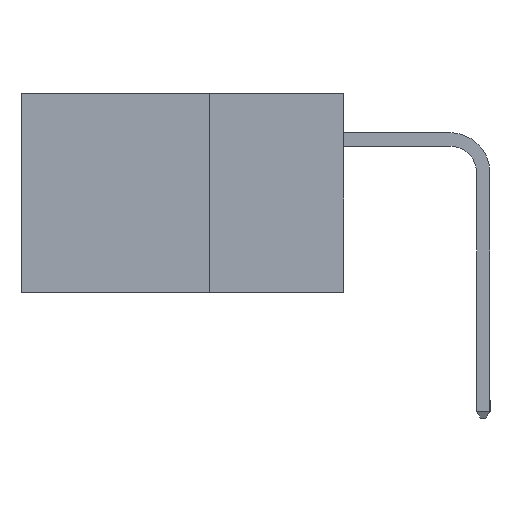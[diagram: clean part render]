
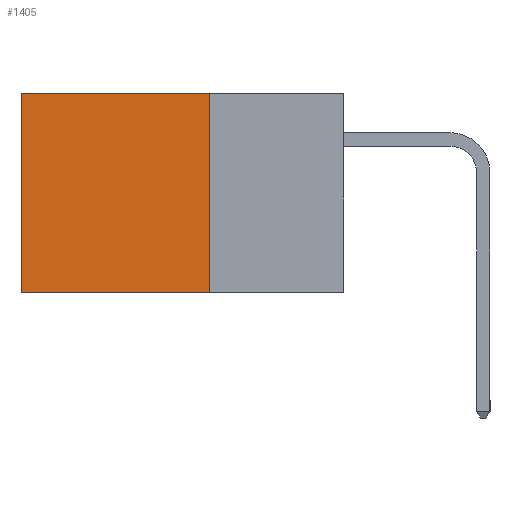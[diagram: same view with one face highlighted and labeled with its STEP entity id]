
A CAD part, left-side view. The second image highlights one B-rep face of the part: STEP entity #1405.
In plain terms, the highlighted planar face has unit normal (-1, 0, 0).
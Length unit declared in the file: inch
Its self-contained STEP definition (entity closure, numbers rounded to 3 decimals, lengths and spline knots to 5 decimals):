
#421 = VERTEX_POINT ( 'NONE', #11745 ) ;
#1313 = DIRECTION ( 'NONE',  ( 1., 0., 0. ) ) ;
#1405 = ADVANCED_FACE ( 'NONE', ( #15971 ), #9843, .F. ) ;
#2176 = VERTEX_POINT ( 'NONE', #10069 ) ;
#2707 = VECTOR ( 'NONE', #11695, 39.37008 ) ;
#3219 = LINE ( 'NONE', #14516, #14065 ) ;
#3481 = DIRECTION ( 'NONE',  ( 0., 1., 0. ) ) ;
#5278 = VECTOR ( 'NONE', #3481, 39.37008 ) ;
#5578 = CARTESIAN_POINT ( 'NONE',  ( 0.2615, 0.25, -0.37 ) ) ;
#5884 = ORIENTED_EDGE ( 'NONE', *, *, #10088, .F. ) ;
#6276 = CARTESIAN_POINT ( 'NONE',  ( 0.2615, 0.25, 0. ) ) ;
#6612 = ORIENTED_EDGE ( 'NONE', *, *, #6989, .T. ) ;
#6844 = EDGE_LOOP ( 'NONE', ( #7627, #5884, #12613, #6612 ) ) ;
#6989 = EDGE_CURVE ( 'NONE', #2176, #421, #12816, .T. ) ;
#7627 = ORIENTED_EDGE ( 'NONE', *, *, #11199, .T. ) ;
#7789 = VECTOR ( 'NONE', #15414, 39.37008 ) ;
#8059 = EDGE_CURVE ( 'NONE', #2176, #14943, #3219, .T. ) ;
#8375 = VERTEX_POINT ( 'NONE', #9587 ) ;
#9587 = CARTESIAN_POINT ( 'NONE',  ( 0.2615, 0.6, -0.37 ) ) ;
#9788 = CARTESIAN_POINT ( 'NONE',  ( 0.2615, 0.6, -0.37 ) ) ;
#9835 = LINE ( 'NONE', #10259, #2707 ) ;
#9843 = PLANE ( 'NONE',  #17042 ) ;
#10069 = CARTESIAN_POINT ( 'NONE',  ( 0.2615, 0.25, 0. ) ) ;
#10088 = EDGE_CURVE ( 'NONE', #14943, #8375, #9835, .T. ) ;
#10259 = CARTESIAN_POINT ( 'NONE',  ( 0.2615, 0.25, -0.37 ) ) ;
#11199 = EDGE_CURVE ( 'NONE', #421, #8375, #15271, .T. ) ;
#11261 = DIRECTION ( 'NONE',  ( 0., 0., -1. ) ) ;
#11695 = DIRECTION ( 'NONE',  ( 0., 1., 0. ) ) ;
#11745 = CARTESIAN_POINT ( 'NONE',  ( 0.2615, 0.6, 0. ) ) ;
#12613 = ORIENTED_EDGE ( 'NONE', *, *, #8059, .F. ) ;
#12816 = LINE ( 'NONE', #6276, #5278 ) ;
#14065 = VECTOR ( 'NONE', #15901, 39.37008 ) ;
#14198 = CARTESIAN_POINT ( 'NONE',  ( 0.2615, 0.25, -0.37 ) ) ;
#14516 = CARTESIAN_POINT ( 'NONE',  ( 0.2615, 0.25, -0.37 ) ) ;
#14943 = VERTEX_POINT ( 'NONE', #14198 ) ;
#15271 = LINE ( 'NONE', #9788, #7789 ) ;
#15414 = DIRECTION ( 'NONE',  ( 0., 0., -1. ) ) ;
#15901 = DIRECTION ( 'NONE',  ( 0., 0., -1. ) ) ;
#15971 = FACE_OUTER_BOUND ( 'NONE', #6844, .T. ) ;
#17042 = AXIS2_PLACEMENT_3D ( 'NONE', #5578, #1313, #11261 ) ;
